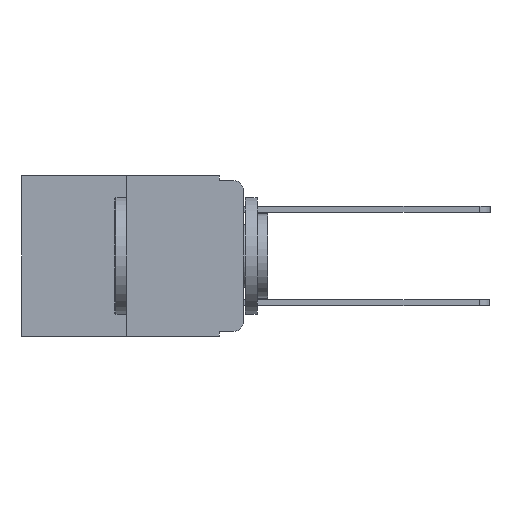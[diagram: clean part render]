
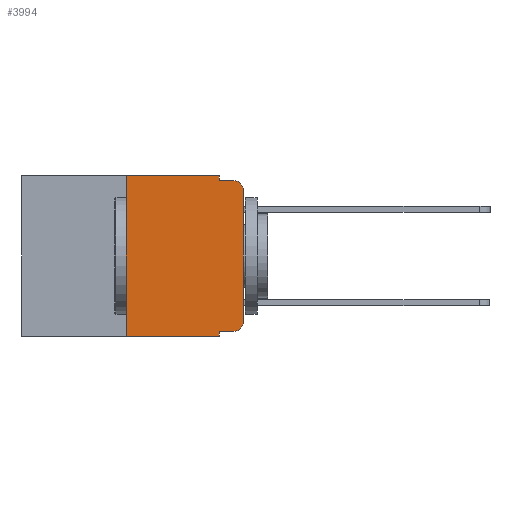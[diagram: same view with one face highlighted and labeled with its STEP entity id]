
A CAD part, left-side view. The second image highlights one B-rep face of the part: STEP entity #3994.
In plain terms, the highlighted planar face has unit normal (-1, 0, 0).
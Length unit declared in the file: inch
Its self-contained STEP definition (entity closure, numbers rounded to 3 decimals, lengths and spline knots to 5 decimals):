
#100 = EDGE_CURVE ( 'NONE', #11697, #17607, #14787, .T. ) ;
#412 = VECTOR ( 'NONE', #12763, 39.37008 ) ;
#859 = ORIENTED_EDGE ( 'NONE', *, *, #5721, .T. ) ;
#1327 = DIRECTION ( 'NONE',  ( 1., 0., 0. ) ) ;
#1969 = DIRECTION ( 'NONE',  ( -1., 0., 0. ) ) ;
#1972 = DIRECTION ( 'NONE',  ( 0., 0., 1. ) ) ;
#2421 = CARTESIAN_POINT ( 'NONE',  ( 0., 0.051, -0.333 ) ) ;
#2540 = CARTESIAN_POINT ( 'NONE',  ( 0., 0.25, 0. ) ) ;
#2542 = CARTESIAN_POINT ( 'NONE',  ( 0., 0.02, -0.01 ) ) ;
#2619 = EDGE_CURVE ( 'NONE', #4374, #3462, #5758, .T. ) ;
#2886 = VECTOR ( 'NONE', #16445, 39.37008 ) ;
#2902 = CARTESIAN_POINT ( 'NONE',  ( 0., 0.473, -0.343 ) ) ;
#2978 = EDGE_CURVE ( 'NONE', #17066, #24358, #19512, .T. ) ;
#3263 = AXIS2_PLACEMENT_3D ( 'NONE', #24340, #1327, #14898 ) ;
#3462 = VERTEX_POINT ( 'NONE', #12376 ) ;
#3649 = CARTESIAN_POINT ( 'NONE',  ( 0., 0.25, 0. ) ) ;
#3790 = DIRECTION ( 'NONE',  ( -1., 0., 0. ) ) ;
#3912 = CIRCLE ( 'NONE', #10315, 0.02 ) ;
#3994 = ADVANCED_FACE ( 'NONE', ( #7252 ), #11017, .F. ) ;
#4004 = CARTESIAN_POINT ( 'NONE',  ( 0., 0.051, -0.333 ) ) ;
#4279 = DIRECTION ( 'NONE',  ( 0., -1., 0. ) ) ;
#4374 = VERTEX_POINT ( 'NONE', #2421 ) ;
#4711 = CARTESIAN_POINT ( 'NONE',  ( 0., 0.051, -0.01 ) ) ;
#5506 = EDGE_LOOP ( 'NONE', ( #19939, #11294, #9025, #13414, #23746, #15234, #24147, #20030, #7455, #859 ) ) ;
#5721 = EDGE_CURVE ( 'NONE', #9091, #24178, #21447, .T. ) ;
#5758 = LINE ( 'NONE', #10936, #412 ) ;
#5974 = DIRECTION ( 'NONE',  ( 0., -1., 0. ) ) ;
#6725 = LINE ( 'NONE', #20701, #21319 ) ;
#6832 = LINE ( 'NONE', #4004, #16406 ) ;
#7252 = FACE_OUTER_BOUND ( 'NONE', #5506, .T. ) ;
#7455 = ORIENTED_EDGE ( 'NONE', *, *, #24852, .T. ) ;
#7570 = CARTESIAN_POINT ( 'NONE',  ( 0., 0.25, -0.343 ) ) ;
#7796 = CARTESIAN_POINT ( 'NONE',  ( 0., 0.051, -0.01 ) ) ;
#8713 = CARTESIAN_POINT ( 'NONE',  ( 0., 0., -0.03 ) ) ;
#8949 = VERTEX_POINT ( 'NONE', #8713 ) ;
#8984 = EDGE_CURVE ( 'NONE', #13094, #11697, #13770, .T. ) ;
#9025 = ORIENTED_EDGE ( 'NONE', *, *, #100, .F. ) ;
#9091 = VERTEX_POINT ( 'NONE', #18712 ) ;
#9167 = EDGE_CURVE ( 'NONE', #24178, #8949, #23545, .T. ) ;
#9353 = DIRECTION ( 'NONE',  ( 0., 0., 1. ) ) ;
#9675 = VECTOR ( 'NONE', #4279, 39.37008 ) ;
#10315 = AXIS2_PLACEMENT_3D ( 'NONE', #13593, #1969, #15525 ) ;
#10724 = AXIS2_PLACEMENT_3D ( 'NONE', #15323, #3790, #20391 ) ;
#10936 = CARTESIAN_POINT ( 'NONE',  ( 0., 0.051, 0. ) ) ;
#11017 = PLANE ( 'NONE',  #3263 ) ;
#11294 = ORIENTED_EDGE ( 'NONE', *, *, #22886, .T. ) ;
#11697 = VERTEX_POINT ( 'NONE', #7796 ) ;
#12060 = CARTESIAN_POINT ( 'NONE',  ( 0., 0.051, 0. ) ) ;
#12376 = CARTESIAN_POINT ( 'NONE',  ( 0., 0.051, -0.343 ) ) ;
#12571 = CARTESIAN_POINT ( 'NONE',  ( 0., 0.051, 0. ) ) ;
#12763 = DIRECTION ( 'NONE',  ( 0., 0., -1. ) ) ;
#12868 = LINE ( 'NONE', #2902, #17995 ) ;
#13094 = VERTEX_POINT ( 'NONE', #12060 ) ;
#13414 = ORIENTED_EDGE ( 'NONE', *, *, #8984, .F. ) ;
#13593 = CARTESIAN_POINT ( 'NONE',  ( 0., 0.02, -0.03 ) ) ;
#13770 = LINE ( 'NONE', #12571, #2886 ) ;
#14384 = EDGE_CURVE ( 'NONE', #17066, #3462, #12868, .T. ) ;
#14787 = LINE ( 'NONE', #4711, #9675 ) ;
#14898 = DIRECTION ( 'NONE',  ( 0., 0., -1. ) ) ;
#15234 = ORIENTED_EDGE ( 'NONE', *, *, #2978, .F. ) ;
#15323 = CARTESIAN_POINT ( 'NONE',  ( 0., 0.02, -0.313 ) ) ;
#15525 = DIRECTION ( 'NONE',  ( 0., 0., -1. ) ) ;
#16406 = VECTOR ( 'NONE', #5974, 39.37008 ) ;
#16445 = DIRECTION ( 'NONE',  ( 0., 0., -1. ) ) ;
#17066 = VERTEX_POINT ( 'NONE', #7570 ) ;
#17607 = VERTEX_POINT ( 'NONE', #2542 ) ;
#17995 = VECTOR ( 'NONE', #18336, 39.37008 ) ;
#18336 = DIRECTION ( 'NONE',  ( 0., -1., 0. ) ) ;
#18579 = VECTOR ( 'NONE', #9353, 39.37008 ) ;
#18712 = CARTESIAN_POINT ( 'NONE',  ( 0., 0.02, -0.333 ) ) ;
#18931 = VECTOR ( 'NONE', #1972, 39.37008 ) ;
#19512 = LINE ( 'NONE', #2540, #18931 ) ;
#19939 = ORIENTED_EDGE ( 'NONE', *, *, #9167, .T. ) ;
#20030 = ORIENTED_EDGE ( 'NONE', *, *, #2619, .F. ) ;
#20391 = DIRECTION ( 'NONE',  ( 0., 0., -1. ) ) ;
#20701 = CARTESIAN_POINT ( 'NONE',  ( 0., 0.473, 0. ) ) ;
#21319 = VECTOR ( 'NONE', #24487, 39.37008 ) ;
#21447 = CIRCLE ( 'NONE', #10724, 0.02 ) ;
#22096 = EDGE_CURVE ( 'NONE', #24358, #13094, #6725, .T. ) ;
#22886 = EDGE_CURVE ( 'NONE', #8949, #17607, #3912, .T. ) ;
#23545 = LINE ( 'NONE', #24436, #18579 ) ;
#23746 = ORIENTED_EDGE ( 'NONE', *, *, #22096, .F. ) ;
#24049 = CARTESIAN_POINT ( 'NONE',  ( 0., 0., -0.313 ) ) ;
#24147 = ORIENTED_EDGE ( 'NONE', *, *, #14384, .T. ) ;
#24178 = VERTEX_POINT ( 'NONE', #24049 ) ;
#24340 = CARTESIAN_POINT ( 'NONE',  ( 0., 0.473, 0. ) ) ;
#24358 = VERTEX_POINT ( 'NONE', #3649 ) ;
#24436 = CARTESIAN_POINT ( 'NONE',  ( 0., 0., 0. ) ) ;
#24487 = DIRECTION ( 'NONE',  ( 0., -1., 0. ) ) ;
#24852 = EDGE_CURVE ( 'NONE', #4374, #9091, #6832, .T. ) ;
